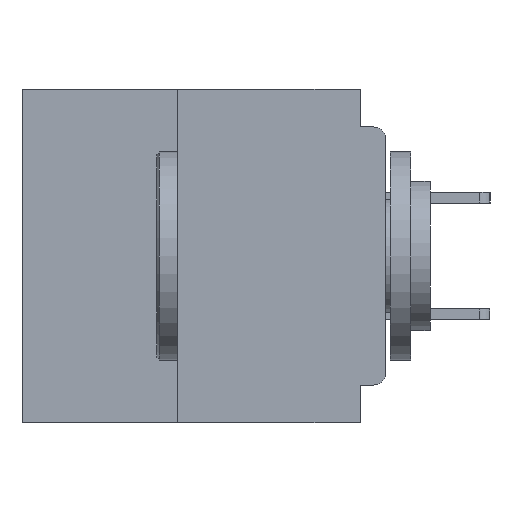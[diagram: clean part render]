
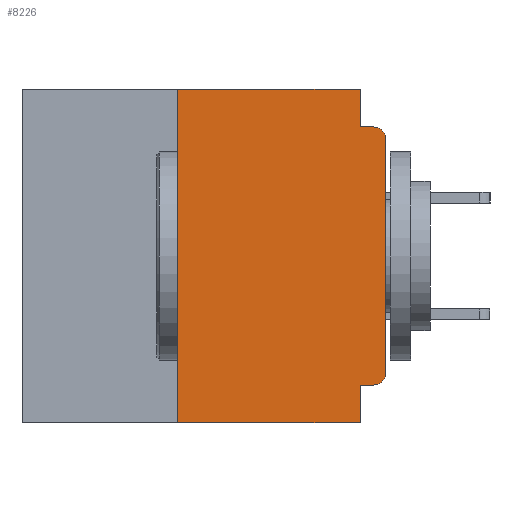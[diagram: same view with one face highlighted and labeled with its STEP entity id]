
A CAD part, left-side view. The second image highlights one B-rep face of the part: STEP entity #8226.
In plain terms, the highlighted planar face has unit normal (-1, 0, 0).
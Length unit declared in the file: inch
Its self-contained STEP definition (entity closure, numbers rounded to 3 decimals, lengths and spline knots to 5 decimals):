
#181 = CARTESIAN_POINT ( 'NONE',  ( 0., 0.031, -0.4 ) ) ;
#229 = EDGE_CURVE ( 'NONE', #28713, #19599, #36254, .T. ) ;
#339 = CARTESIAN_POINT ( 'NONE',  ( 0., 0.437, 0. ) ) ;
#455 = DIRECTION ( 'NONE',  ( 0., 0., -1. ) ) ;
#550 = CARTESIAN_POINT ( 'NONE',  ( 0., 0., -0.06 ) ) ;
#841 = VERTEX_POINT ( 'NONE', #20856 ) ;
#1109 = VECTOR ( 'NONE', #2576, 39.37008 ) ;
#2576 = DIRECTION ( 'NONE',  ( 0., 1., 0. ) ) ;
#2822 = CARTESIAN_POINT ( 'NONE',  ( 0., 0., -0.34 ) ) ;
#3338 = VECTOR ( 'NONE', #455, 39.37008 ) ;
#4057 = LINE ( 'NONE', #14036, #11367 ) ;
#4499 = CIRCLE ( 'NONE', #14131, 0.015 ) ;
#4677 = EDGE_CURVE ( 'NONE', #19310, #38898, #10798, .T. ) ;
#4779 = ORIENTED_EDGE ( 'NONE', *, *, #24941, .T. ) ;
#4827 = EDGE_CURVE ( 'NONE', #841, #27110, #29663, .T. ) ;
#5275 = VECTOR ( 'NONE', #7040, 39.37008 ) ;
#6095 = CARTESIAN_POINT ( 'NONE',  ( 0., 0.25, -0.4 ) ) ;
#6137 = EDGE_CURVE ( 'NONE', #27110, #23587, #16804, .T. ) ;
#6377 = DIRECTION ( 'NONE',  ( -1., 0., 0. ) ) ;
#7040 = DIRECTION ( 'NONE',  ( 0., 0., 1. ) ) ;
#7720 = ORIENTED_EDGE ( 'NONE', *, *, #21479, .F. ) ;
#7766 = CARTESIAN_POINT ( 'NONE',  ( 0., 0.25, 0. ) ) ;
#7852 = CARTESIAN_POINT ( 'NONE',  ( 0., 0.031, -0.4 ) ) ;
#8226 = ADVANCED_FACE ( 'NONE', ( #13214 ), #10862, .F. ) ;
#9745 = DIRECTION ( 'NONE',  ( 0., -1., 0. ) ) ;
#10213 = EDGE_CURVE ( 'NONE', #17359, #18940, #38130, .T. ) ;
#10798 = LINE ( 'NONE', #18580, #34448 ) ;
#10862 = PLANE ( 'NONE',  #27502 ) ;
#11367 = VECTOR ( 'NONE', #32548, 39.37008 ) ;
#13214 = FACE_OUTER_BOUND ( 'NONE', #17634, .T. ) ;
#13287 = CARTESIAN_POINT ( 'NONE',  ( 0., 0.25, -0.4 ) ) ;
#13732 = VERTEX_POINT ( 'NONE', #29766 ) ;
#14036 = CARTESIAN_POINT ( 'NONE',  ( 0., 0.437, -0.4 ) ) ;
#14131 = AXIS2_PLACEMENT_3D ( 'NONE', #24915, #6377, #28025 ) ;
#15442 = ORIENTED_EDGE ( 'NONE', *, *, #4677, .F. ) ;
#15555 = VECTOR ( 'NONE', #23520, 39.37008 ) ;
#16129 = LINE ( 'NONE', #339, #38746 ) ;
#16804 = LINE ( 'NONE', #37443, #32252 ) ;
#17096 = DIRECTION ( 'NONE',  ( 1., 0., 0. ) ) ;
#17359 = VERTEX_POINT ( 'NONE', #6095 ) ;
#17632 = LINE ( 'NONE', #39566, #1109 ) ;
#17634 = EDGE_LOOP ( 'NONE', ( #33264, #20739, #15442, #35694, #22732, #28527, #4779, #23232, #7720, #33341 ) ) ;
#18442 = DIRECTION ( 'NONE',  ( 0., -1., 0. ) ) ;
#18580 = CARTESIAN_POINT ( 'NONE',  ( 0., 0., -0.045 ) ) ;
#18940 = VERTEX_POINT ( 'NONE', #7766 ) ;
#19003 = DIRECTION ( 'NONE',  ( 0., 0., 1. ) ) ;
#19310 = VERTEX_POINT ( 'NONE', #21957 ) ;
#19599 = VERTEX_POINT ( 'NONE', #7852 ) ;
#20739 = ORIENTED_EDGE ( 'NONE', *, *, #21595, .T. ) ;
#20856 = CARTESIAN_POINT ( 'NONE',  ( 0., 0.015, -0.355 ) ) ;
#21479 = EDGE_CURVE ( 'NONE', #841, #28713, #17632, .T. ) ;
#21595 = EDGE_CURVE ( 'NONE', #23587, #38898, #4499, .T. ) ;
#21957 = CARTESIAN_POINT ( 'NONE',  ( 0., 0.031, -0.045 ) ) ;
#22162 = EDGE_CURVE ( 'NONE', #18940, #13732, #16129, .T. ) ;
#22666 = CARTESIAN_POINT ( 'NONE',  ( 0., 0.031, -0.355 ) ) ;
#22732 = ORIENTED_EDGE ( 'NONE', *, *, #22162, .F. ) ;
#23193 = EDGE_CURVE ( 'NONE', #13732, #19310, #23782, .T. ) ;
#23232 = ORIENTED_EDGE ( 'NONE', *, *, #229, .F. ) ;
#23520 = DIRECTION ( 'NONE',  ( 0., 0., -1. ) ) ;
#23587 = VERTEX_POINT ( 'NONE', #550 ) ;
#23782 = LINE ( 'NONE', #32667, #15555 ) ;
#24333 = AXIS2_PLACEMENT_3D ( 'NONE', #39515, #39433, #39351 ) ;
#24915 = CARTESIAN_POINT ( 'NONE',  ( 0., 0.015, -0.06 ) ) ;
#24941 = EDGE_CURVE ( 'NONE', #17359, #19599, #4057, .T. ) ;
#27110 = VERTEX_POINT ( 'NONE', #2822 ) ;
#27502 = AXIS2_PLACEMENT_3D ( 'NONE', #35546, #17096, #38611 ) ;
#28025 = DIRECTION ( 'NONE',  ( 0., 0., -1. ) ) ;
#28527 = ORIENTED_EDGE ( 'NONE', *, *, #10213, .F. ) ;
#28713 = VERTEX_POINT ( 'NONE', #22666 ) ;
#29663 = CIRCLE ( 'NONE', #24333, 0.015 ) ;
#29766 = CARTESIAN_POINT ( 'NONE',  ( 0., 0.031, 0. ) ) ;
#32252 = VECTOR ( 'NONE', #19003, 39.37008 ) ;
#32548 = DIRECTION ( 'NONE',  ( 0., -1., 0. ) ) ;
#32667 = CARTESIAN_POINT ( 'NONE',  ( 0., 0.031, 0. ) ) ;
#33264 = ORIENTED_EDGE ( 'NONE', *, *, #6137, .T. ) ;
#33341 = ORIENTED_EDGE ( 'NONE', *, *, #4827, .T. ) ;
#34448 = VECTOR ( 'NONE', #18442, 39.37008 ) ;
#35546 = CARTESIAN_POINT ( 'NONE',  ( 0., 0.437, 0. ) ) ;
#35555 = CARTESIAN_POINT ( 'NONE',  ( 0., 0.015, -0.045 ) ) ;
#35694 = ORIENTED_EDGE ( 'NONE', *, *, #23193, .F. ) ;
#36254 = LINE ( 'NONE', #181, #3338 ) ;
#37443 = CARTESIAN_POINT ( 'NONE',  ( 0., 0., 0. ) ) ;
#38130 = LINE ( 'NONE', #13287, #5275 ) ;
#38611 = DIRECTION ( 'NONE',  ( 0., 0., -1. ) ) ;
#38746 = VECTOR ( 'NONE', #9745, 39.37008 ) ;
#38898 = VERTEX_POINT ( 'NONE', #35555 ) ;
#39351 = DIRECTION ( 'NONE',  ( 0., 0., -1. ) ) ;
#39433 = DIRECTION ( 'NONE',  ( -1., 0., 0. ) ) ;
#39515 = CARTESIAN_POINT ( 'NONE',  ( 0., 0.015, -0.34 ) ) ;
#39566 = CARTESIAN_POINT ( 'NONE',  ( 0., 0., -0.355 ) ) ;
